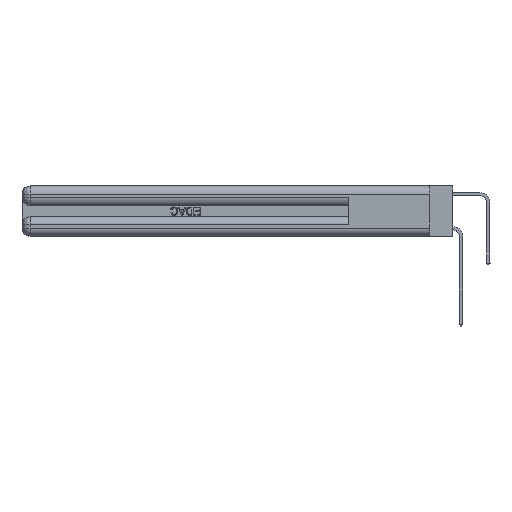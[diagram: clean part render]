
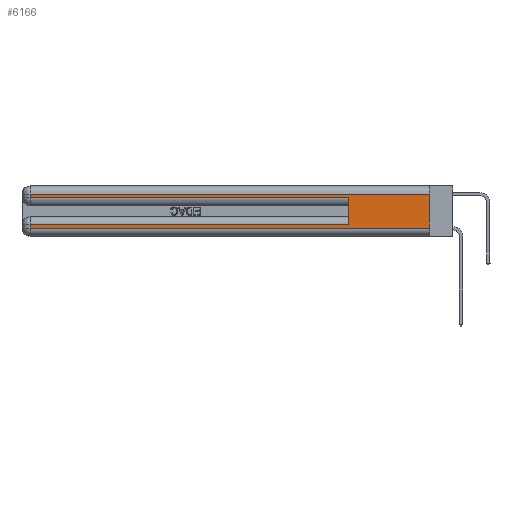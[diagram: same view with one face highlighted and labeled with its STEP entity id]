
A CAD part, left-side view. The second image highlights one B-rep face of the part: STEP entity #6166.
In plain terms, the highlighted planar face has unit normal (-1, 0, 0).
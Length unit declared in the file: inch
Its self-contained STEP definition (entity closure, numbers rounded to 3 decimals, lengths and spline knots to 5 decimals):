
#149 = DIRECTION ( 'NONE',  ( 0., -1., 0. ) ) ;
#516 = DIRECTION ( 'NONE',  ( 0., 0., -1. ) ) ;
#545 = VERTEX_POINT ( 'NONE', #3889 ) ;
#749 = EDGE_CURVE ( 'NONE', #29125, #16695, #26826, .T. ) ;
#1218 = CARTESIAN_POINT ( 'NONE',  ( 0., 0.6, 0.085 ) ) ;
#1228 = CARTESIAN_POINT ( 'NONE',  ( 0., 2.94, 0.37 ) ) ;
#1383 = CARTESIAN_POINT ( 'NONE',  ( 0., 0., 0.31 ) ) ;
#2170 = CARTESIAN_POINT ( 'NONE',  ( 0., 0., 0.37 ) ) ;
#2779 = ORIENTED_EDGE ( 'NONE', *, *, #749, .T. ) ;
#3506 = VERTEX_POINT ( 'NONE', #17055 ) ;
#3889 = CARTESIAN_POINT ( 'NONE',  ( 0., 0., 0.06 ) ) ;
#4373 = DIRECTION ( 'NONE',  ( 0., 1., 0. ) ) ;
#4539 = AXIS2_PLACEMENT_3D ( 'NONE', #2170, #4806, #12194 ) ;
#4562 = DIRECTION ( 'NONE',  ( 0., 0., -1. ) ) ;
#4806 = DIRECTION ( 'NONE',  ( 1., 0., 0. ) ) ;
#5180 = CARTESIAN_POINT ( 'NONE',  ( 0., 2.94, 0.06 ) ) ;
#5438 = ORIENTED_EDGE ( 'NONE', *, *, #32242, .F. ) ;
#5628 = LINE ( 'NONE', #12677, #21346 ) ;
#6166 = ADVANCED_FACE ( 'NONE', ( #26631 ), #29541, .F. ) ;
#7030 = VECTOR ( 'NONE', #149, 39.37008 ) ;
#7109 = EDGE_CURVE ( 'NONE', #29125, #12056, #9988, .T. ) ;
#7902 = LINE ( 'NONE', #29662, #7030 ) ;
#9247 = VERTEX_POINT ( 'NONE', #16329 ) ;
#9988 = LINE ( 'NONE', #32087, #18247 ) ;
#11222 = ORIENTED_EDGE ( 'NONE', *, *, #7109, .F. ) ;
#11622 = CARTESIAN_POINT ( 'NONE',  ( 0., 0., 0.085 ) ) ;
#11693 = ORIENTED_EDGE ( 'NONE', *, *, #19980, .T. ) ;
#12056 = VERTEX_POINT ( 'NONE', #24211 ) ;
#12194 = DIRECTION ( 'NONE',  ( 0., 0., -1. ) ) ;
#12401 = ORIENTED_EDGE ( 'NONE', *, *, #32006, .T. ) ;
#12677 = CARTESIAN_POINT ( 'NONE',  ( 0., 2.94, 0.37 ) ) ;
#12725 = ORIENTED_EDGE ( 'NONE', *, *, #22499, .T. ) ;
#12958 = VECTOR ( 'NONE', #18549, 39.37008 ) ;
#13046 = EDGE_LOOP ( 'NONE', ( #5438, #11693, #20583, #12725, #11222, #2779, #21699, #12401 ) ) ;
#13317 = VERTEX_POINT ( 'NONE', #26494 ) ;
#13572 = CARTESIAN_POINT ( 'NONE',  ( 0., 2.94, 0.085 ) ) ;
#13871 = LINE ( 'NONE', #1228, #19214 ) ;
#16329 = CARTESIAN_POINT ( 'NONE',  ( 0., 2.94, 0.31 ) ) ;
#16330 = DIRECTION ( 'NONE',  ( 0., 1., 0. ) ) ;
#16695 = VERTEX_POINT ( 'NONE', #13572 ) ;
#17055 = CARTESIAN_POINT ( 'NONE',  ( 0., 0., 0.31 ) ) ;
#18247 = VECTOR ( 'NONE', #19670, 39.37008 ) ;
#18549 = DIRECTION ( 'NONE',  ( 0., -1., 0. ) ) ;
#18642 = LINE ( 'NONE', #1383, #19643 ) ;
#19214 = VECTOR ( 'NONE', #23882, 39.37008 ) ;
#19643 = VECTOR ( 'NONE', #16330, 39.37008 ) ;
#19670 = DIRECTION ( 'NONE',  ( 0., 0., 1. ) ) ;
#19980 = EDGE_CURVE ( 'NONE', #3506, #9247, #18642, .T. ) ;
#20583 = ORIENTED_EDGE ( 'NONE', *, *, #21141, .T. ) ;
#20679 = LINE ( 'NONE', #30629, #12958 ) ;
#21141 = EDGE_CURVE ( 'NONE', #9247, #13317, #13871, .T. ) ;
#21346 = VECTOR ( 'NONE', #516, 39.37008 ) ;
#21699 = ORIENTED_EDGE ( 'NONE', *, *, #23853, .T. ) ;
#22499 = EDGE_CURVE ( 'NONE', #13317, #12056, #20679, .T. ) ;
#23853 = EDGE_CURVE ( 'NONE', #16695, #31123, #5628, .T. ) ;
#23882 = DIRECTION ( 'NONE',  ( 0., 0., -1. ) ) ;
#24211 = CARTESIAN_POINT ( 'NONE',  ( 0., 0.6, 0.285 ) ) ;
#24825 = VECTOR ( 'NONE', #4562, 39.37008 ) ;
#26494 = CARTESIAN_POINT ( 'NONE',  ( 0., 2.94, 0.285 ) ) ;
#26631 = FACE_OUTER_BOUND ( 'NONE', #13046, .T. ) ;
#26826 = LINE ( 'NONE', #11622, #27355 ) ;
#27005 = CARTESIAN_POINT ( 'NONE',  ( 0., 0., 0.37 ) ) ;
#27355 = VECTOR ( 'NONE', #4373, 39.37008 ) ;
#29125 = VERTEX_POINT ( 'NONE', #1218 ) ;
#29465 = LINE ( 'NONE', #27005, #24825 ) ;
#29541 = PLANE ( 'NONE',  #4539 ) ;
#29662 = CARTESIAN_POINT ( 'NONE',  ( 0., 0., 0.06 ) ) ;
#30629 = CARTESIAN_POINT ( 'NONE',  ( 0., 0., 0.285 ) ) ;
#31123 = VERTEX_POINT ( 'NONE', #5180 ) ;
#32006 = EDGE_CURVE ( 'NONE', #31123, #545, #7902, .T. ) ;
#32087 = CARTESIAN_POINT ( 'NONE',  ( 0., 0.6, 0.145 ) ) ;
#32242 = EDGE_CURVE ( 'NONE', #3506, #545, #29465, .T. ) ;
